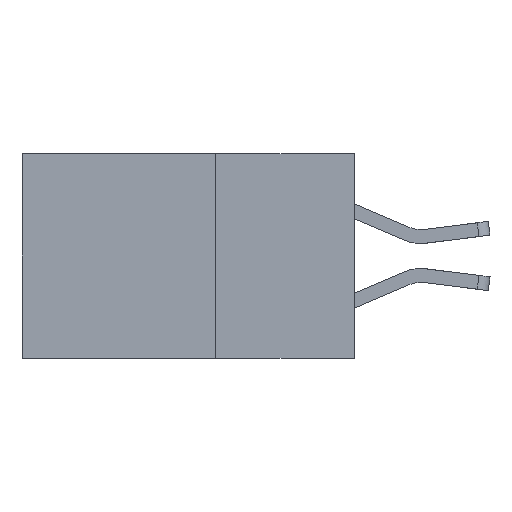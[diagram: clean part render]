
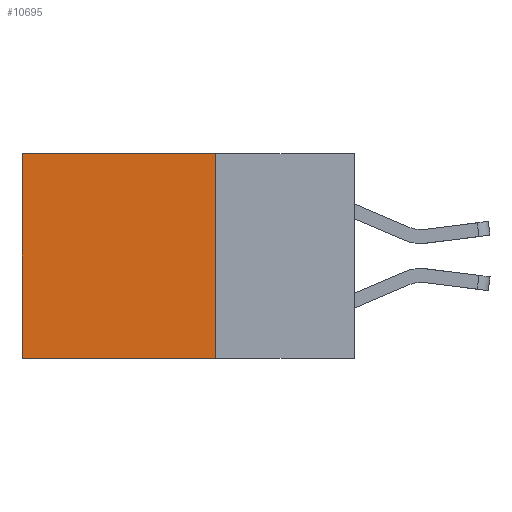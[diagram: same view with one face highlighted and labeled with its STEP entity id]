
A CAD part, left-side view. The second image highlights one B-rep face of the part: STEP entity #10695.
In plain terms, the highlighted planar face has unit normal (-1, 0, 0).
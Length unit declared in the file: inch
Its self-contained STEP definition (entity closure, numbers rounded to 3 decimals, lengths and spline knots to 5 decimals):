
#246 = CARTESIAN_POINT ( 'NONE',  ( 0.298, 0.25, -0.37 ) ) ;
#547 = ORIENTED_EDGE ( 'NONE', *, *, #8828, .T. ) ;
#628 = CARTESIAN_POINT ( 'NONE',  ( 0.298, 0.6, 0. ) ) ;
#1090 = CARTESIAN_POINT ( 'NONE',  ( 0.298, 0.6, 0. ) ) ;
#1167 = VECTOR ( 'NONE', #8048, 39.37008 ) ;
#1257 = VERTEX_POINT ( 'NONE', #5391 ) ;
#1434 = CARTESIAN_POINT ( 'NONE',  ( 0.298, 0.25, 0. ) ) ;
#2091 = ORIENTED_EDGE ( 'NONE', *, *, #8381, .F. ) ;
#2398 = DIRECTION ( 'NONE',  ( 0., 0., -1. ) ) ;
#2998 = EDGE_LOOP ( 'NONE', ( #3536, #7391, #2091, #547 ) ) ;
#3376 = LINE ( 'NONE', #9074, #1167 ) ;
#3536 = ORIENTED_EDGE ( 'NONE', *, *, #6285, .T. ) ;
#4241 = LINE ( 'NONE', #11422, #11440 ) ;
#5391 = CARTESIAN_POINT ( 'NONE',  ( 0.298, 0.6, -0.37 ) ) ;
#6109 = DIRECTION ( 'NONE',  ( 0., 1., 0. ) ) ;
#6285 = EDGE_CURVE ( 'NONE', #11385, #1257, #7995, .T. ) ;
#6535 = DIRECTION ( 'NONE',  ( 0., 0., -1. ) ) ;
#6573 = DIRECTION ( 'NONE',  ( 1., 0., 0. ) ) ;
#6729 = VERTEX_POINT ( 'NONE', #246 ) ;
#6733 = PLANE ( 'NONE',  #10842 ) ;
#7114 = LINE ( 'NONE', #10078, #9752 ) ;
#7286 = CARTESIAN_POINT ( 'NONE',  ( 0.298, 0.25, 0. ) ) ;
#7391 = ORIENTED_EDGE ( 'NONE', *, *, #7613, .F. ) ;
#7613 = EDGE_CURVE ( 'NONE', #6729, #1257, #4241, .T. ) ;
#7995 = LINE ( 'NONE', #628, #9416 ) ;
#8048 = DIRECTION ( 'NONE',  ( 0., 1., 0. ) ) ;
#8369 = VERTEX_POINT ( 'NONE', #7286 ) ;
#8381 = EDGE_CURVE ( 'NONE', #8369, #6729, #7114, .T. ) ;
#8828 = EDGE_CURVE ( 'NONE', #8369, #11385, #3376, .T. ) ;
#9074 = CARTESIAN_POINT ( 'NONE',  ( 0.298, 0.25, 0. ) ) ;
#9416 = VECTOR ( 'NONE', #2398, 39.37008 ) ;
#9752 = VECTOR ( 'NONE', #6535, 39.37008 ) ;
#10078 = CARTESIAN_POINT ( 'NONE',  ( 0.298, 0.25, 0. ) ) ;
#10695 = ADVANCED_FACE ( 'NONE', ( #10824 ), #6733, .F. ) ;
#10824 = FACE_OUTER_BOUND ( 'NONE', #2998, .T. ) ;
#10842 = AXIS2_PLACEMENT_3D ( 'NONE', #1434, #6573, #11114 ) ;
#11114 = DIRECTION ( 'NONE',  ( 0., 0., -1. ) ) ;
#11385 = VERTEX_POINT ( 'NONE', #1090 ) ;
#11422 = CARTESIAN_POINT ( 'NONE',  ( 0.298, 0.25, -0.37 ) ) ;
#11440 = VECTOR ( 'NONE', #6109, 39.37008 ) ;
